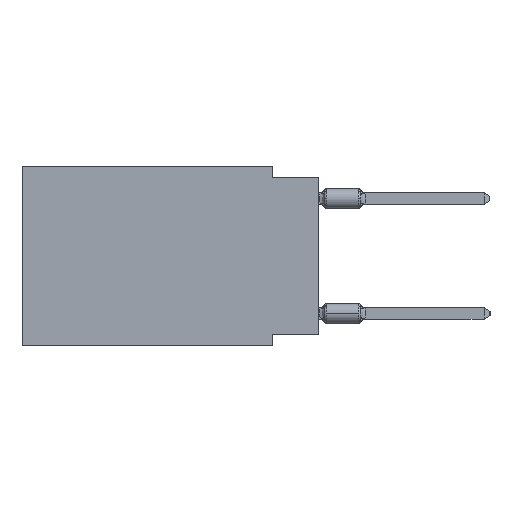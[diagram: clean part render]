
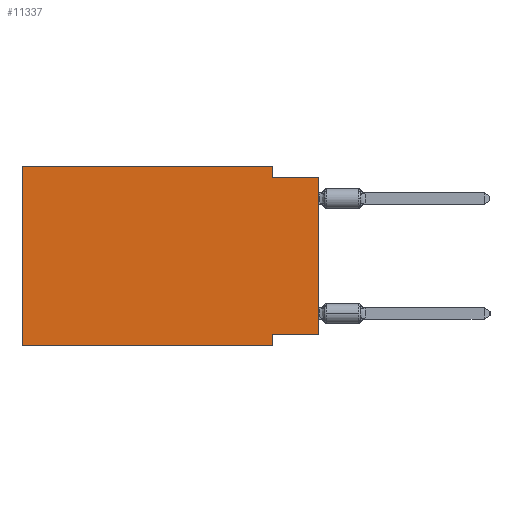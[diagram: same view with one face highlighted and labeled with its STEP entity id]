
A CAD part, left-side view. The second image highlights one B-rep face of the part: STEP entity #11337.
In plain terms, the highlighted planar face has unit normal (-1, 0, 0).
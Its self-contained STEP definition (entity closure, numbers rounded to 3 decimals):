
#153 = ORIENTED_EDGE ( 'NONE', *, *, #8667, .F. ) ;
#551 = DIRECTION ( 'NONE',  ( 0., -1., 0. ) ) ;
#694 = EDGE_CURVE ( 'NONE', #23733, #40426, #10497, .T. ) ;
#1950 = EDGE_LOOP ( 'NONE', ( #2178, #33938, #10353, #12395, #28736, #12340, #153, #5123 ) ) ;
#2178 = ORIENTED_EDGE ( 'NONE', *, *, #694, .T. ) ;
#2423 = CARTESIAN_POINT ( 'NONE',  ( 0., 2.54, 0. ) ) ;
#2823 = VECTOR ( 'NONE', #19220, 1000. ) ;
#4627 = DIRECTION ( 'NONE',  ( 0., 0., 1. ) ) ;
#5123 = ORIENTED_EDGE ( 'NONE', *, *, #22511, .F. ) ;
#6792 = VECTOR ( 'NONE', #4627, 1000. ) ;
#6987 = CARTESIAN_POINT ( 'NONE',  ( 0., 0., -0.635 ) ) ;
#7377 = CARTESIAN_POINT ( 'NONE',  ( 0., 16.383, -9.906 ) ) ;
#7518 = CARTESIAN_POINT ( 'NONE',  ( 0., 0., -0.635 ) ) ;
#8093 = CARTESIAN_POINT ( 'NONE',  ( 0., 2.54, -9.906 ) ) ;
#8151 = EDGE_CURVE ( 'NONE', #34934, #14649, #10067, .T. ) ;
#8416 = VECTOR ( 'NONE', #20753, 1000. ) ;
#8460 = CARTESIAN_POINT ( 'NONE',  ( 0., 16.383, 0. ) ) ;
#8512 = CARTESIAN_POINT ( 'NONE',  ( 0., 0., -9.271 ) ) ;
#8659 = DIRECTION ( 'NONE',  ( 1., 0., 0. ) ) ;
#8667 = EDGE_CURVE ( 'NONE', #35369, #25782, #36505, .T. ) ;
#10067 = LINE ( 'NONE', #38276, #15665 ) ;
#10353 = ORIENTED_EDGE ( 'NONE', *, *, #17627, .F. ) ;
#10497 = LINE ( 'NONE', #11119, #26954 ) ;
#10702 = DIRECTION ( 'NONE',  ( 0., 0., 1. ) ) ;
#11119 = CARTESIAN_POINT ( 'NONE',  ( 0., 0., 0. ) ) ;
#11337 = ADVANCED_FACE ( 'NONE', ( #21323 ), #12180, .F. ) ;
#12180 = PLANE ( 'NONE',  #14506 ) ;
#12340 = ORIENTED_EDGE ( 'NONE', *, *, #27512, .T. ) ;
#12395 = ORIENTED_EDGE ( 'NONE', *, *, #8151, .F. ) ;
#14506 = AXIS2_PLACEMENT_3D ( 'NONE', #8460, #8659, #33969 ) ;
#14649 = VERTEX_POINT ( 'NONE', #34747 ) ;
#15665 = VECTOR ( 'NONE', #35589, 1000. ) ;
#15935 = VECTOR ( 'NONE', #551, 1000. ) ;
#16454 = CARTESIAN_POINT ( 'NONE',  ( 0., 2.54, -9.271 ) ) ;
#17627 = EDGE_CURVE ( 'NONE', #14649, #37904, #27731, .T. ) ;
#19220 = DIRECTION ( 'NONE',  ( 0., -1., 0. ) ) ;
#19818 = CARTESIAN_POINT ( 'NONE',  ( 0., 16.383, -9.906 ) ) ;
#19985 = LINE ( 'NONE', #32625, #6792 ) ;
#20677 = CARTESIAN_POINT ( 'NONE',  ( 0., 2.54, -9.906 ) ) ;
#20753 = DIRECTION ( 'NONE',  ( 0., 0., -1. ) ) ;
#21323 = FACE_OUTER_BOUND ( 'NONE', #1950, .T. ) ;
#22511 = EDGE_CURVE ( 'NONE', #23733, #35369, #26140, .T. ) ;
#23135 = EDGE_CURVE ( 'NONE', #37904, #40426, #35190, .T. ) ;
#23733 = VERTEX_POINT ( 'NONE', #8512 ) ;
#24606 = DIRECTION ( 'NONE',  ( 0., 0., -1. ) ) ;
#25782 = VERTEX_POINT ( 'NONE', #20677 ) ;
#26056 = VERTEX_POINT ( 'NONE', #19818 ) ;
#26140 = LINE ( 'NONE', #29669, #39747 ) ;
#26849 = EDGE_CURVE ( 'NONE', #26056, #34934, #19985, .T. ) ;
#26954 = VECTOR ( 'NONE', #10702, 1000. ) ;
#27512 = EDGE_CURVE ( 'NONE', #26056, #25782, #34971, .T. ) ;
#27731 = LINE ( 'NONE', #2423, #34742 ) ;
#28736 = ORIENTED_EDGE ( 'NONE', *, *, #26849, .F. ) ;
#29669 = CARTESIAN_POINT ( 'NONE',  ( 0., 0., -9.271 ) ) ;
#32625 = CARTESIAN_POINT ( 'NONE',  ( 0., 16.383, 0. ) ) ;
#33938 = ORIENTED_EDGE ( 'NONE', *, *, #23135, .F. ) ;
#33969 = DIRECTION ( 'NONE',  ( 0., 0., -1. ) ) ;
#34742 = VECTOR ( 'NONE', #24606, 1000. ) ;
#34747 = CARTESIAN_POINT ( 'NONE',  ( 0., 2.54, 0. ) ) ;
#34934 = VERTEX_POINT ( 'NONE', #38883 ) ;
#34971 = LINE ( 'NONE', #7377, #2823 ) ;
#35190 = LINE ( 'NONE', #6987, #15935 ) ;
#35369 = VERTEX_POINT ( 'NONE', #16454 ) ;
#35589 = DIRECTION ( 'NONE',  ( 0., -1., 0. ) ) ;
#36005 = CARTESIAN_POINT ( 'NONE',  ( 0., 2.54, -0.635 ) ) ;
#36505 = LINE ( 'NONE', #8093, #8416 ) ;
#37904 = VERTEX_POINT ( 'NONE', #36005 ) ;
#38276 = CARTESIAN_POINT ( 'NONE',  ( 0., 16.383, 0. ) ) ;
#38360 = DIRECTION ( 'NONE',  ( 0., 1., 0. ) ) ;
#38883 = CARTESIAN_POINT ( 'NONE',  ( 0., 16.383, 0. ) ) ;
#39747 = VECTOR ( 'NONE', #38360, 1000. ) ;
#40426 = VERTEX_POINT ( 'NONE', #7518 ) ;
